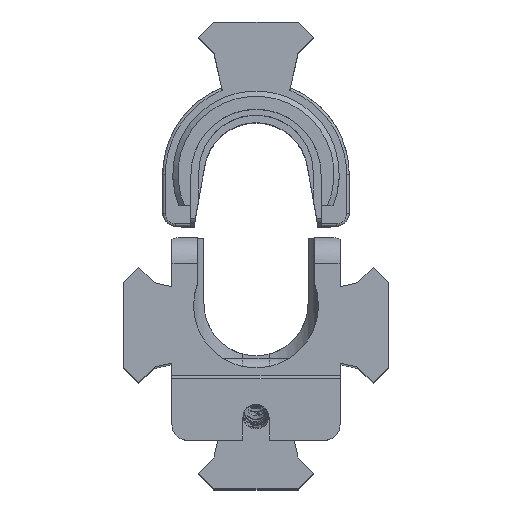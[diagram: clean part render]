
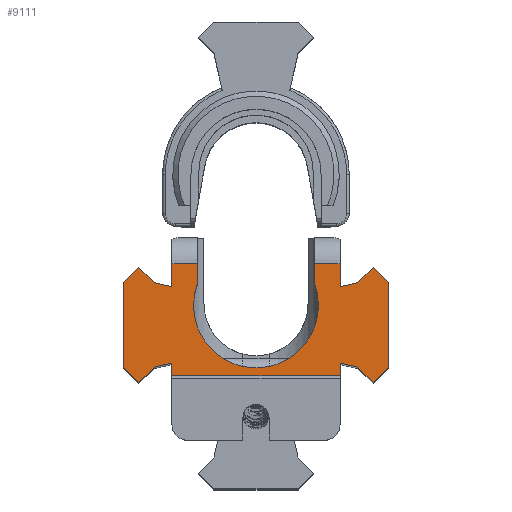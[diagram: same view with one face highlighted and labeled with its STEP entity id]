
A CAD part, top view. The second image highlights one B-rep face of the part: STEP entity #9111.
In plain terms, the highlighted planar face has unit normal (0, 0, 1).
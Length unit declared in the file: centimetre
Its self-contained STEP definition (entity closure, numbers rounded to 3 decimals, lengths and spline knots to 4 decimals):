
#156=LINE($,#13009,#1214);
#164=LINE($,#13756,#1222);
#171=LINE($,#13773,#1229);
#203=LINE($,#13837,#1261);
#212=LINE($,#13855,#1270);
#215=LINE($,#13861,#1273);
#380=LINE($,#14191,#1438);
#383=LINE($,#14208,#1441);
#387=LINE($,#14215,#1445);
#542=LINE($,#15198,#1600);
#591=LINE($,#15282,#1649);
#593=LINE($,#15287,#1651);
#596=LINE($,#15292,#1654);
#599=LINE($,#15297,#1657);
#601=LINE($,#15308,#1659);
#603=LINE($,#15317,#1661);
#608=LINE($,#15362,#1666);
#629=LINE($,#16857,#1687);
#673=LINE($,#17405,#1731);
#677=LINE($,#17415,#1735);
#720=LINE($,#17625,#1778);
#740=LINE($,#18161,#1798);
#741=LINE($,#18162,#1799);
#1214=VECTOR($,#9985,0.2415);
#1222=VECTOR($,#9999,0.2417);
#1229=VECTOR($,#10014,0.4138);
#1261=VECTOR($,#10048,0.4138);
#1270=VECTOR($,#10063,1.6225);
#1273=VECTOR($,#10068,0.4138);
#1438=VECTOR($,#10399,0.4138);
#1441=VECTOR($,#10404,0.3504);
#1445=VECTOR($,#10410,0.3504);
#1600=VECTOR($,#10679,0.4138);
#1649=VECTOR($,#10786,0.4138);
#1651=VECTOR($,#10790,0.4138);
#1654=VECTOR($,#10795,0.4138);
#1657=VECTOR($,#10800,1.6225);
#1659=VECTOR($,#10804,0.3505);
#1661=VECTOR($,#10808,0.3505);
#1666=VECTOR($,#10833,0.4391);
#1687=VECTOR($,#10888,0.49);
#1731=VECTOR($,#10990,0.3824);
#1735=VECTOR($,#10998,0.3824);
#1778=VECTOR($,#11163,3.23);
#1798=VECTOR($,#11243,0.49);
#1799=VECTOR($,#11244,0.4389);
#2494=PLANE($,#9687);
#2978=FACE_OUTER_BOUND($,#3509,.T.);
#3509=EDGE_LOOP($,(#7578,#7579,#7580,#7581,#7582,#7583,#7584,#7585,#7586,
#7587,#7588,#7589,#7590,#7591,#7592,#7593,#7594,#7595,#7596,#7597,#7598,
#7599,#7600,#7601));
#3896=CIRCLE($,#9593,1.2);
#3987=VERTEX_POINT($,#13006);
#3988=VERTEX_POINT($,#13008);
#4011=VERTEX_POINT($,#13753);
#4012=VERTEX_POINT($,#13755);
#4017=VERTEX_POINT($,#13771);
#4018=VERTEX_POINT($,#13772);
#4049=VERTEX_POINT($,#13836);
#4055=VERTEX_POINT($,#13854);
#4057=VERTEX_POINT($,#13860);
#4139=VERTEX_POINT($,#14190);
#4144=VERTEX_POINT($,#14212);
#4259=VERTEX_POINT($,#15196);
#4260=VERTEX_POINT($,#15197);
#4266=VERTEX_POINT($,#15281);
#4267=VERTEX_POINT($,#15285);
#4268=VERTEX_POINT($,#15286);
#4269=VERTEX_POINT($,#15291);
#4273=VERTEX_POINT($,#15314);
#4288=VERTEX_POINT($,#15360);
#4321=VERTEX_POINT($,#16855);
#4370=VERTEX_POINT($,#17332);
#4371=VERTEX_POINT($,#17334);
#4381=VERTEX_POINT($,#17413);
#4444=VERTEX_POINT($,#18160);
#4809=EDGE_CURVE($,#3987,#3988,#156,.T.);
#4841=EDGE_CURVE($,#4011,#4012,#164,.T.);
#4849=EDGE_CURVE($,#4017,#4018,#171,.T.);
#4881=EDGE_CURVE($,#4018,#4049,#203,.T.);
#4890=EDGE_CURVE($,#4049,#4055,#212,.T.);
#4893=EDGE_CURVE($,#4055,#4057,#215,.T.);
#5058=EDGE_CURVE($,#4057,#4139,#380,.T.);
#5063=EDGE_CURVE($,#4012,#4017,#383,.T.);
#5067=EDGE_CURVE($,#4139,#4144,#387,.T.);
#5225=EDGE_CURVE($,#4259,#4260,#542,.T.);
#5274=EDGE_CURVE($,#4266,#4259,#591,.T.);
#5276=EDGE_CURVE($,#4267,#4268,#593,.T.);
#5279=EDGE_CURVE($,#4269,#4267,#596,.T.);
#5282=EDGE_CURVE($,#4268,#4266,#599,.T.);
#5285=EDGE_CURVE($,#4260,#3987,#601,.T.);
#5288=EDGE_CURVE($,#4273,#4269,#603,.T.);
#5304=EDGE_CURVE($,#4288,#4273,#608,.T.);
#5354=EDGE_CURVE($,#4288,#4321,#629,.T.);
#5423=EDGE_CURVE($,#4370,#4371,#3896,.T.);
#5431=EDGE_CURVE($,#4371,#4321,#673,.T.);
#5436=EDGE_CURVE($,#4381,#4370,#677,.T.);
#5517=EDGE_CURVE($,#3988,#4011,#720,.T.);
#5554=EDGE_CURVE($,#4381,#4444,#740,.T.);
#5555=EDGE_CURVE($,#4144,#4444,#741,.T.);
#7578=ORIENTED_EDGE($,*,*,#5304,.F.);
#7579=ORIENTED_EDGE($,*,*,#5354,.T.);
#7580=ORIENTED_EDGE($,*,*,#5431,.F.);
#7581=ORIENTED_EDGE($,*,*,#5423,.F.);
#7582=ORIENTED_EDGE($,*,*,#5436,.F.);
#7583=ORIENTED_EDGE($,*,*,#5554,.T.);
#7584=ORIENTED_EDGE($,*,*,#5555,.F.);
#7585=ORIENTED_EDGE($,*,*,#5067,.F.);
#7586=ORIENTED_EDGE($,*,*,#5058,.F.);
#7587=ORIENTED_EDGE($,*,*,#4893,.F.);
#7588=ORIENTED_EDGE($,*,*,#4890,.F.);
#7589=ORIENTED_EDGE($,*,*,#4881,.F.);
#7590=ORIENTED_EDGE($,*,*,#4849,.F.);
#7591=ORIENTED_EDGE($,*,*,#5063,.F.);
#7592=ORIENTED_EDGE($,*,*,#4841,.F.);
#7593=ORIENTED_EDGE($,*,*,#5517,.F.);
#7594=ORIENTED_EDGE($,*,*,#4809,.F.);
#7595=ORIENTED_EDGE($,*,*,#5285,.F.);
#7596=ORIENTED_EDGE($,*,*,#5225,.F.);
#7597=ORIENTED_EDGE($,*,*,#5274,.F.);
#7598=ORIENTED_EDGE($,*,*,#5282,.F.);
#7599=ORIENTED_EDGE($,*,*,#5276,.F.);
#7600=ORIENTED_EDGE($,*,*,#5279,.F.);
#7601=ORIENTED_EDGE($,*,*,#5288,.F.);
#9111=ADVANCED_FACE($,(#2978),#2494,.T.);
#9593=AXIS2_PLACEMENT_3D($,#17335,#10985,#10986);
#9687=AXIS2_PLACEMENT_3D($,#18159,#11241,#11242);
#9985=DIRECTION($,(0.,-1.,0.));
#9999=DIRECTION($,(0.,1.,0.));
#10014=DIRECTION($,(-0.71,-0.704,0.));
#10048=DIRECTION($,(-0.71,0.704,0.));
#10063=DIRECTION($,(0.,1.,0.));
#10068=DIRECTION($,(0.71,0.704,0.));
#10399=DIRECTION($,(0.71,-0.704,0.));
#10404=DIRECTION($,(-0.976,-0.218,0.));
#10410=DIRECTION($,(0.976,-0.218,0.));
#10679=DIRECTION($,(-0.71,0.704,0.));
#10786=DIRECTION($,(-0.71,-0.704,0.));
#10790=DIRECTION($,(0.71,-0.704,0.));
#10795=DIRECTION($,(0.71,0.704,0.));
#10800=DIRECTION($,(0.,-1.,0.));
#10804=DIRECTION($,(-0.976,0.218,0.));
#10808=DIRECTION($,(0.976,0.218,0.));
#10833=DIRECTION($,(0.,-1.,0.));
#10888=DIRECTION($,(-1.,0.,0.));
#10985=DIRECTION('center_axis',(0.,0.,
1.));
#10986=DIRECTION('ref_axis',(1.,0.,0.));
#10990=DIRECTION($,(0.,1.,0.));
#10998=DIRECTION($,(0.,-1.,0.));
#11163=DIRECTION($,(-1.,0.,0.));
#11241=DIRECTION('center_axis',(0.,0.,
1.));
#11242=DIRECTION('ref_axis',(1.,0.,0.));
#11243=DIRECTION($,(-1.,0.,0.));
#11244=DIRECTION($,(0.,1.,0.));
#13006=CARTESIAN_POINT('',(1.575,-1.7009,-0.16));
#13008=CARTESIAN_POINT('',(1.575,-1.9424,-0.16));
#13009=CARTESIAN_POINT($,(1.575,-2.3283,-0.16));
#13753=CARTESIAN_POINT('',(-1.655,-1.9424,-0.16));
#13755=CARTESIAN_POINT('',(-1.655,-1.7007,-0.16));
#13756=CARTESIAN_POINT($,(-1.655,-2.3283,-0.16));
#13771=CARTESIAN_POINT('',(-1.9969,-1.7773,-0.16));
#13772=CARTESIAN_POINT('',(-2.2909,-2.0685,-0.16));
#13773=CARTESIAN_POINT($,(0.004,0.2048,-0.16));
#13836=CARTESIAN_POINT('',(-2.5849,-1.7773,-0.16));
#13837=CARTESIAN_POINT($,(-3.1771,-1.1906,-0.16));
#13854=CARTESIAN_POINT('',(-2.5849,-0.1547,-0.16));
#13855=CARTESIAN_POINT($,(-2.5849,1.517,-0.16));
#13860=CARTESIAN_POINT('',(-2.2909,0.1365,-0.16));
#13861=CARTESIAN_POINT($,(-0.6943,1.7181,-0.16));
#14190=CARTESIAN_POINT('',(-1.9969,-0.1547,-0.16));
#14191=CARTESIAN_POINT($,(-2.4789,0.3227,-0.16));
#14208=CARTESIAN_POINT($,(-0.162,-1.3665,-0.16));
#14212=CARTESIAN_POINT('',(-1.655,-0.2313,-0.16));
#14215=CARTESIAN_POINT($,(-1.2207,-0.3285,-0.16));
#15196=CARTESIAN_POINT('',(2.211,-2.0687,-0.16));
#15197=CARTESIAN_POINT('',(1.917,-1.7774,-0.16));
#15198=CARTESIAN_POINT($,(0.1886,-0.0653,-0.16));
#15281=CARTESIAN_POINT('',(2.505,-1.7774,-0.16));
#15282=CARTESIAN_POINT($,(3.3698,-0.9208,-0.16));
#15285=CARTESIAN_POINT('',(2.211,0.1363,-0.16));
#15286=CARTESIAN_POINT('',(2.505,-0.1549,-0.16));
#15287=CARTESIAN_POINT($,(0.8868,1.448,-0.16));
#15291=CARTESIAN_POINT('',(1.917,-0.1549,-0.16));
#15292=CARTESIAN_POINT($,(2.6716,0.5926,-0.16));
#15297=CARTESIAN_POINT($,(2.505,1.5169,-0.16));
#15308=CARTESIAN_POINT($,(0.5963,-1.4818,-0.16));
#15314=CARTESIAN_POINT('',(1.575,-0.2315,-0.16));
#15317=CARTESIAN_POINT($,(1.655,-0.2136,-0.16));
#15360=CARTESIAN_POINT('',(1.575,0.2076,-0.16));
#15362=CARTESIAN_POINT($,(1.575,-2.3283,-0.16));
#16855=CARTESIAN_POINT('',(1.085,0.2076,-0.16));
#16857=CARTESIAN_POINT($,(1.76,0.2076,-0.16));
#17332=CARTESIAN_POINT('',(-1.165,-0.1748,-0.16));
#17334=CARTESIAN_POINT('',(1.085,-0.1748,-0.16));
#17335=CARTESIAN_POINT('Origin',(-0.04,-0.5924,
-0.16));
#17405=CARTESIAN_POINT($,(1.085,-0.1748,-0.16));
#17413=CARTESIAN_POINT('',(-1.165,0.2076,-0.16));
#17415=CARTESIAN_POINT($,(-1.165,0.2076,-0.16));
#17625=CARTESIAN_POINT($,(1.575,-1.9424,-0.16));
#18159=CARTESIAN_POINT('Origin',(-1.39,-2.9424,-0.16));
#18160=CARTESIAN_POINT('',(-1.655,0.2076,-0.16));
#18161=CARTESIAN_POINT($,(-1.165,0.2076,-0.16));
#18162=CARTESIAN_POINT($,(-1.655,-2.3283,-0.16));
